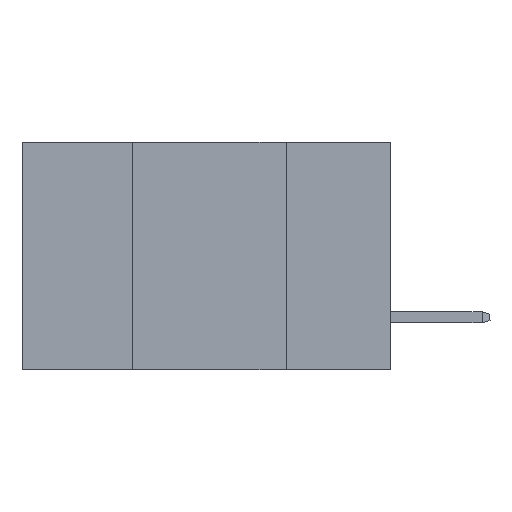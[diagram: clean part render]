
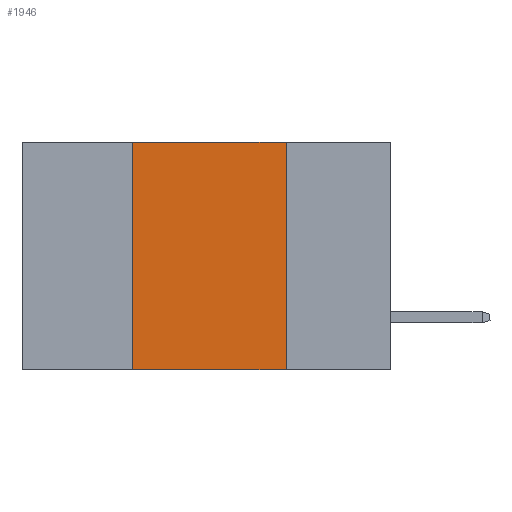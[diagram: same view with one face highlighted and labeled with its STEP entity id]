
A CAD part, left-side view. The second image highlights one B-rep face of the part: STEP entity #1946.
In plain terms, the highlighted planar face has unit normal (-1, 0, 0).
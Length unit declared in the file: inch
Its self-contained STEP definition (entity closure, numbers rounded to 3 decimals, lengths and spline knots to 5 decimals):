
#14 = ORIENTED_EDGE ( 'NONE', *, *, #2431, .F. ) ;
#21 = FACE_OUTER_BOUND ( 'NONE', #6400, .T. ) ;
#91 = PLANE ( 'NONE',  #507 ) ;
#506 = EDGE_CURVE ( 'NONE', #5619, #1168, #5512, .T. ) ;
#507 = AXIS2_PLACEMENT_3D ( 'NONE', #2665, #1913, #1751 ) ;
#1168 = VERTEX_POINT ( 'NONE', #10473 ) ;
#1322 = EDGE_CURVE ( 'NONE', #2341, #1168, #11316, .T. ) ;
#1406 = CARTESIAN_POINT ( 'NONE',  ( 0., 0.42, 0. ) ) ;
#1566 = CARTESIAN_POINT ( 'NONE',  ( 0., 0.42, -0.37 ) ) ;
#1751 = DIRECTION ( 'NONE',  ( 0., 0., -1. ) ) ;
#1913 = DIRECTION ( 'NONE',  ( 1., 0., 0. ) ) ;
#1922 = VECTOR ( 'NONE', #9267, 39.37008 ) ;
#1946 = ADVANCED_FACE ( 'NONE', ( #21 ), #91, .F. ) ;
#2341 = VERTEX_POINT ( 'NONE', #1566 ) ;
#2431 = EDGE_CURVE ( 'NONE', #8402, #5619, #10929, .T. ) ;
#2515 = ORIENTED_EDGE ( 'NONE', *, *, #3450, .F. ) ;
#2665 = CARTESIAN_POINT ( 'NONE',  ( 0., 0.6, 0. ) ) ;
#3050 = LINE ( 'NONE', #1406, #5464 ) ;
#3450 = EDGE_CURVE ( 'NONE', #2341, #8402, #3050, .T. ) ;
#4303 = DIRECTION ( 'NONE',  ( 0., 0., -1. ) ) ;
#4321 = CARTESIAN_POINT ( 'NONE',  ( 0., 0.17, 0. ) ) ;
#5401 = CARTESIAN_POINT ( 'NONE',  ( 0., 0.17, 0. ) ) ;
#5464 = VECTOR ( 'NONE', #8501, 39.37008 ) ;
#5512 = LINE ( 'NONE', #4321, #5784 ) ;
#5619 = VERTEX_POINT ( 'NONE', #5401 ) ;
#5784 = VECTOR ( 'NONE', #4303, 39.37008 ) ;
#6400 = EDGE_LOOP ( 'NONE', ( #6990, #14, #2515, #9531 ) ) ;
#6885 = VECTOR ( 'NONE', #10635, 39.37008 ) ;
#6990 = ORIENTED_EDGE ( 'NONE', *, *, #506, .F. ) ;
#8402 = VERTEX_POINT ( 'NONE', #9290 ) ;
#8501 = DIRECTION ( 'NONE',  ( 0., 0., 1. ) ) ;
#9267 = DIRECTION ( 'NONE',  ( 0., -1., 0. ) ) ;
#9290 = CARTESIAN_POINT ( 'NONE',  ( 0., 0.42, 0. ) ) ;
#9531 = ORIENTED_EDGE ( 'NONE', *, *, #1322, .T. ) ;
#9611 = CARTESIAN_POINT ( 'NONE',  ( 0., 0.6, 0. ) ) ;
#10473 = CARTESIAN_POINT ( 'NONE',  ( 0., 0.17, -0.37 ) ) ;
#10635 = DIRECTION ( 'NONE',  ( 0., -1., 0. ) ) ;
#10677 = CARTESIAN_POINT ( 'NONE',  ( 0., 0.6, -0.37 ) ) ;
#10929 = LINE ( 'NONE', #9611, #1922 ) ;
#11316 = LINE ( 'NONE', #10677, #6885 ) ;
